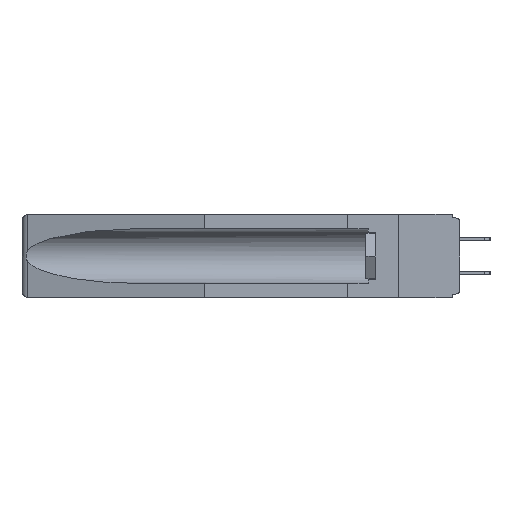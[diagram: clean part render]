
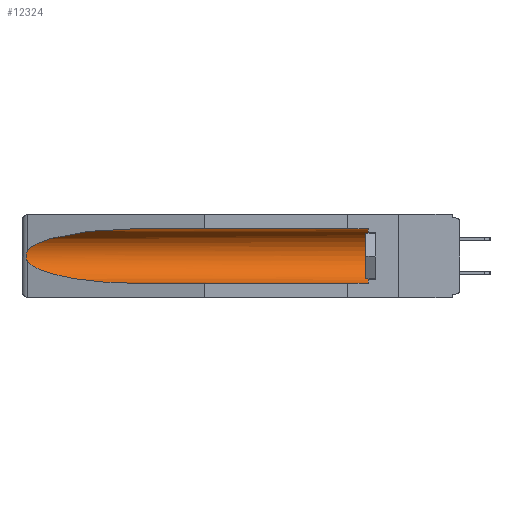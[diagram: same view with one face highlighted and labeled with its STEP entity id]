
A CAD part, left-side view. The second image highlights one B-rep face of the part: STEP entity #12324.
In plain terms, the highlighted cylindrical face has radius 2.857 mm (diameter 5.715 mm), a partial arc.
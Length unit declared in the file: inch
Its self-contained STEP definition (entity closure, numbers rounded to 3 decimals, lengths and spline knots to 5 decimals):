
#121 = DIRECTION ( 'NONE',  ( 0., 0., 1. ) ) ;
#927 = ORIENTED_EDGE ( 'NONE', *, *, #9497, .T. ) ;
#1096 = ORIENTED_EDGE ( 'NONE', *, *, #12949, .T. ) ;
#1104 = CARTESIAN_POINT ( 'NONE',  ( 0.155, -0.30754, -0.059 ) ) ;
#1157 = CARTESIAN_POINT ( 'NONE',  ( 0.25451, 1.48313, -0.24835 ) ) ;
#3062 = CARTESIAN_POINT ( 'NONE',  ( 0.155, 0.126, -0.059 ) ) ;
#3226 = CYLINDRICAL_SURFACE ( 'NONE', #19707, 0.1125 ) ;
#3962 = ORIENTED_EDGE ( 'NONE', *, *, #6480, .T. ) ;
#4622 = ORIENTED_EDGE ( 'NONE', *, *, #17850, .T. ) ;
#5410 = CARTESIAN_POINT ( 'NONE',  ( 0.26537, 1.52718, -0.19328 ) ) ;
#5576 = CARTESIAN_POINT ( 'NONE',  ( 0.26655, 1.53094, -0.18657 ) ) ;
#5593 = EDGE_LOOP ( 'NONE', ( #1096, #927, #4622, #18846, #12543, #3962 ) ) ;
#5728 = AXIS2_PLACEMENT_3D ( 'NONE', #17756, #17840, #12065 ) ;
#6364 = CARTESIAN_POINT ( 'NONE',  ( 0.26537, 1.52718, -0.14972 ) ) ;
#6480 = EDGE_CURVE ( 'NONE', #12234, #24376, #9451, .T. ) ;
#6853 =( BOUNDED_CURVE ( )  B_SPLINE_CURVE ( 3, ( #11691, #7888, #15716, #6364 ),
 .UNSPECIFIED., .F., .F. ) 
 B_SPLINE_CURVE_WITH_KNOTS ( ( 4, 4 ),
 ( 4.71239, 6.08839 ),
 .UNSPECIFIED. ) 
 CURVE ( )  GEOMETRIC_REPRESENTATION_ITEM ( )  RATIONAL_B_SPLINE_CURVE ( ( 1., 0.848, 0.848, 1. ) ) 
 REPRESENTATION_ITEM ( '' )  );
#7179 =( BOUNDED_CURVE ( )  B_SPLINE_CURVE ( 3, ( #10592, #1157, #8771, #16863 ),
 .UNSPECIFIED., .F., .F. ) 
 B_SPLINE_CURVE_WITH_KNOTS ( ( 4, 4 ),
 ( 0.1948, 1.5708 ),
 .UNSPECIFIED. ) 
 CURVE ( )  GEOMETRIC_REPRESENTATION_ITEM ( )  RATIONAL_B_SPLINE_CURVE ( ( 1., 0.848, 0.848, 1. ) ) 
 REPRESENTATION_ITEM ( '' )  );
#7405 = CARTESIAN_POINT ( 'NONE',  ( 0.2675, 1.53308, -0.17534 ) ) ;
#7799 = VERTEX_POINT ( 'NONE', #5410 ) ;
#7888 = CARTESIAN_POINT ( 'NONE',  ( 0.21114, 1.30732, -0.059 ) ) ;
#8771 = CARTESIAN_POINT ( 'NONE',  ( 0.21114, 1.30732, -0.284 ) ) ;
#9414 = VERTEX_POINT ( 'NONE', #21331 ) ;
#9451 = LINE ( 'NONE', #1104, #23186 ) ;
#9476 = CARTESIAN_POINT ( 'NONE',  ( 0.26597, 1.52961, -0.15275 ) ) ;
#9497 = EDGE_CURVE ( 'NONE', #23653, #7799, #16020, .T. ) ;
#10592 = CARTESIAN_POINT ( 'NONE',  ( 0.26537, 1.52718, -0.19328 ) ) ;
#11691 = CARTESIAN_POINT ( 'NONE',  ( 0.155, 1.07973, -0.059 ) ) ;
#12065 = DIRECTION ( 'NONE',  ( 0., 0., 1. ) ) ;
#12234 = VERTEX_POINT ( 'NONE', #3062 ) ;
#12324 = ADVANCED_FACE ( 'NONE', ( #17239 ), #3226, .F. ) ;
#12346 = LINE ( 'NONE', #23625, #21617 ) ;
#12543 = ORIENTED_EDGE ( 'NONE', *, *, #16982, .T. ) ;
#12949 = EDGE_CURVE ( 'NONE', #24376, #23653, #6853, .T. ) ;
#12964 = CARTESIAN_POINT ( 'NONE',  ( 0.2675, 1.53308, -0.16763 ) ) ;
#13789 = EDGE_CURVE ( 'NONE', #9414, #16739, #12346, .T. ) ;
#15016 = CARTESIAN_POINT ( 'NONE',  ( 0.155, 1.07973, -0.284 ) ) ;
#15530 = CARTESIAN_POINT ( 'NONE',  ( 0.26537, 1.52718, -0.14972 ) ) ;
#15716 = CARTESIAN_POINT ( 'NONE',  ( 0.25451, 1.48313, -0.09465 ) ) ;
#16020 = B_SPLINE_CURVE_WITH_KNOTS ( 'NONE', 3,
 ( #20599, #9476, #18847, #22833, #12964, #7405, #22668, #5576, #24501, #24740 ),
 .UNSPECIFIED., .F., .F.,
 ( 4, 2, 2, 2, 4 ),
 ( 0., 0.00029, 0.00058, 0.00087, 0.00117 ),
 .UNSPECIFIED. ) ;
#16739 = VERTEX_POINT ( 'NONE', #15016 ) ;
#16863 = CARTESIAN_POINT ( 'NONE',  ( 0.155, 1.07973, -0.284 ) ) ;
#16982 = EDGE_CURVE ( 'NONE', #9414, #12234, #19261, .T. ) ;
#17239 = FACE_OUTER_BOUND ( 'NONE', #5593, .T. ) ;
#17427 = CARTESIAN_POINT ( 'NONE',  ( 0.155, -0.30754, -0.1715 ) ) ;
#17756 = CARTESIAN_POINT ( 'NONE',  ( 0.155, 0.126, -0.1715 ) ) ;
#17840 = DIRECTION ( 'NONE',  ( 0., -1., 0. ) ) ;
#17850 = EDGE_CURVE ( 'NONE', #7799, #16739, #7179, .T. ) ;
#18237 = DIRECTION ( 'NONE',  ( 0., 1., 0. ) ) ;
#18846 = ORIENTED_EDGE ( 'NONE', *, *, #13789, .F. ) ;
#18847 = CARTESIAN_POINT ( 'NONE',  ( 0.26654, 1.53092, -0.15636 ) ) ;
#19261 = CIRCLE ( 'NONE', #5728, 0.1125 ) ;
#19263 = DIRECTION ( 'NONE',  ( 0., 1., 0. ) ) ;
#19707 = AXIS2_PLACEMENT_3D ( 'NONE', #17427, #19263, #121 ) ;
#20599 = CARTESIAN_POINT ( 'NONE',  ( 0.26537, 1.52718, -0.14972 ) ) ;
#21331 = CARTESIAN_POINT ( 'NONE',  ( 0.155, 0.126, -0.284 ) ) ;
#21617 = VECTOR ( 'NONE', #23462, 39.37008 ) ;
#22668 = CARTESIAN_POINT ( 'NONE',  ( 0.2673, 1.53269, -0.17917 ) ) ;
#22833 = CARTESIAN_POINT ( 'NONE',  ( 0.2673, 1.5327, -0.16383 ) ) ;
#23186 = VECTOR ( 'NONE', #18237, 39.37008 ) ;
#23462 = DIRECTION ( 'NONE',  ( 0., 1., 0. ) ) ;
#23625 = CARTESIAN_POINT ( 'NONE',  ( 0.155, -0.30754, -0.284 ) ) ;
#23653 = VERTEX_POINT ( 'NONE', #15530 ) ;
#24376 = VERTEX_POINT ( 'NONE', #24496 ) ;
#24496 = CARTESIAN_POINT ( 'NONE',  ( 0.155, 1.07973, -0.059 ) ) ;
#24501 = CARTESIAN_POINT ( 'NONE',  ( 0.26597, 1.5296, -0.19026 ) ) ;
#24740 = CARTESIAN_POINT ( 'NONE',  ( 0.26537, 1.52718, -0.19328 ) ) ;
